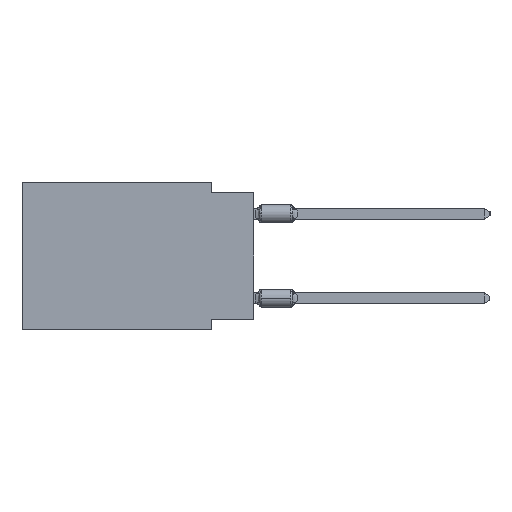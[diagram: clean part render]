
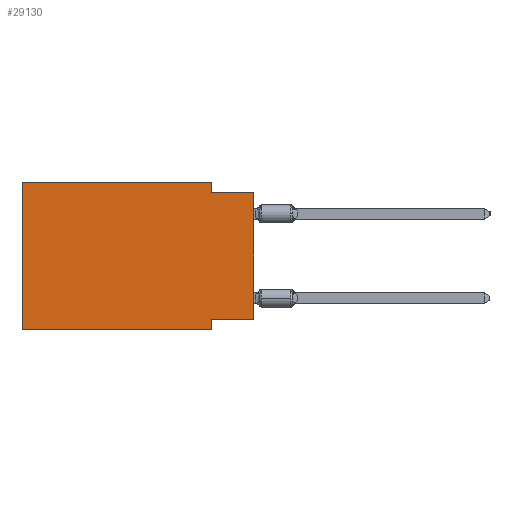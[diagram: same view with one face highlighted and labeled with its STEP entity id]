
A CAD part, left-side view. The second image highlights one B-rep face of the part: STEP entity #29130.
In plain terms, the highlighted planar face has unit normal (-1, 0, 0).
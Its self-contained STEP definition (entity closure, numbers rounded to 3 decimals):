
#166 = EDGE_CURVE ( 'NONE', #42037, #4223, #9251, .T. ) ;
#1439 = PLANE ( 'NONE',  #3843 ) ;
#1578 = CARTESIAN_POINT ( 'NONE',  ( 0., 2.54, -8.255 ) ) ;
#3093 = VERTEX_POINT ( 'NONE', #22915 ) ;
#3843 = AXIS2_PLACEMENT_3D ( 'NONE', #4085, #16096, #15376 ) ;
#4085 = CARTESIAN_POINT ( 'NONE',  ( 0., 13.97, 0. ) ) ;
#4223 = VERTEX_POINT ( 'NONE', #11890 ) ;
#4360 = CARTESIAN_POINT ( 'NONE',  ( 0., 13.97, -8.89 ) ) ;
#4601 = EDGE_CURVE ( 'NONE', #4223, #26962, #32955, .T. ) ;
#4646 = DIRECTION ( 'NONE',  ( 0., 0., -1. ) ) ;
#4659 = EDGE_CURVE ( 'NONE', #46856, #40781, #15416, .T. ) ;
#5146 = CARTESIAN_POINT ( 'NONE',  ( 0., 2.54, -0.635 ) ) ;
#5626 = ORIENTED_EDGE ( 'NONE', *, *, #14805, .T. ) ;
#5647 = CARTESIAN_POINT ( 'NONE',  ( 0., 13.97, 0. ) ) ;
#6246 = CARTESIAN_POINT ( 'NONE',  ( 0., 0., -8.255 ) ) ;
#8059 = DIRECTION ( 'NONE',  ( 0., 0., 1. ) ) ;
#8736 = CARTESIAN_POINT ( 'NONE',  ( 0., 0., -0.635 ) ) ;
#8811 = DIRECTION ( 'NONE',  ( 0., 1., 0. ) ) ;
#9219 = LINE ( 'NONE', #41877, #9990 ) ;
#9251 = LINE ( 'NONE', #5647, #9334 ) ;
#9334 = VECTOR ( 'NONE', #10193, 1000. ) ;
#9573 = VECTOR ( 'NONE', #8059, 1000. ) ;
#9990 = VECTOR ( 'NONE', #4646, 1000. ) ;
#10193 = DIRECTION ( 'NONE',  ( 0., -1., 0. ) ) ;
#11890 = CARTESIAN_POINT ( 'NONE',  ( 0., 2.54, 0. ) ) ;
#12707 = VECTOR ( 'NONE', #35850, 1000. ) ;
#13657 = EDGE_CURVE ( 'NONE', #46856, #42037, #27011, .T. ) ;
#14805 = EDGE_CURVE ( 'NONE', #45793, #3093, #21216, .T. ) ;
#15376 = DIRECTION ( 'NONE',  ( 0., 0., -1. ) ) ;
#15416 = LINE ( 'NONE', #4360, #24406 ) ;
#16015 = LINE ( 'NONE', #41706, #35792 ) ;
#16096 = DIRECTION ( 'NONE',  ( 1., 0., 0. ) ) ;
#17731 = CARTESIAN_POINT ( 'NONE',  ( 0., 2.54, -8.89 ) ) ;
#19027 = DIRECTION ( 'NONE',  ( 0., -1., 0. ) ) ;
#19299 = LINE ( 'NONE', #8736, #23186 ) ;
#20312 = CARTESIAN_POINT ( 'NONE',  ( 0., 13.97, -8.89 ) ) ;
#20636 = ORIENTED_EDGE ( 'NONE', *, *, #31377, .F. ) ;
#21091 = EDGE_LOOP ( 'NONE', ( #5626, #20636, #29914, #36823, #41711, #24439, #24792, #32752 ) ) ;
#21216 = LINE ( 'NONE', #46661, #12707 ) ;
#22915 = CARTESIAN_POINT ( 'NONE',  ( 0., 0., -0.635 ) ) ;
#23186 = VECTOR ( 'NONE', #45222, 1000. ) ;
#23298 = CARTESIAN_POINT ( 'NONE',  ( 0., 13.97, 0. ) ) ;
#24406 = VECTOR ( 'NONE', #19027, 1000. ) ;
#24439 = ORIENTED_EDGE ( 'NONE', *, *, #4659, .T. ) ;
#24792 = ORIENTED_EDGE ( 'NONE', *, *, #35862, .F. ) ;
#25763 = CARTESIAN_POINT ( 'NONE',  ( 0., 2.54, 0. ) ) ;
#26663 = EDGE_CURVE ( 'NONE', #45793, #32159, #16015, .T. ) ;
#26962 = VERTEX_POINT ( 'NONE', #5146 ) ;
#27011 = LINE ( 'NONE', #41659, #9573 ) ;
#29130 = ADVANCED_FACE ( 'NONE', ( #40602 ), #1439, .F. ) ;
#29914 = ORIENTED_EDGE ( 'NONE', *, *, #4601, .F. ) ;
#31377 = EDGE_CURVE ( 'NONE', #26962, #3093, #19299, .T. ) ;
#32159 = VERTEX_POINT ( 'NONE', #1578 ) ;
#32752 = ORIENTED_EDGE ( 'NONE', *, *, #26663, .F. ) ;
#32955 = LINE ( 'NONE', #25763, #39721 ) ;
#35792 = VECTOR ( 'NONE', #8811, 1000. ) ;
#35850 = DIRECTION ( 'NONE',  ( 0., 0., 1. ) ) ;
#35862 = EDGE_CURVE ( 'NONE', #32159, #40781, #9219, .T. ) ;
#36823 = ORIENTED_EDGE ( 'NONE', *, *, #166, .F. ) ;
#39721 = VECTOR ( 'NONE', #40411, 1000. ) ;
#40411 = DIRECTION ( 'NONE',  ( 0., 0., -1. ) ) ;
#40602 = FACE_OUTER_BOUND ( 'NONE', #21091, .T. ) ;
#40781 = VERTEX_POINT ( 'NONE', #17731 ) ;
#41659 = CARTESIAN_POINT ( 'NONE',  ( 0., 13.97, 0. ) ) ;
#41706 = CARTESIAN_POINT ( 'NONE',  ( 0., 0., -8.255 ) ) ;
#41711 = ORIENTED_EDGE ( 'NONE', *, *, #13657, .F. ) ;
#41877 = CARTESIAN_POINT ( 'NONE',  ( 0., 2.54, -8.89 ) ) ;
#42037 = VERTEX_POINT ( 'NONE', #23298 ) ;
#45222 = DIRECTION ( 'NONE',  ( 0., -1., 0. ) ) ;
#45793 = VERTEX_POINT ( 'NONE', #6246 ) ;
#46661 = CARTESIAN_POINT ( 'NONE',  ( 0., 0., 0. ) ) ;
#46856 = VERTEX_POINT ( 'NONE', #20312 ) ;
